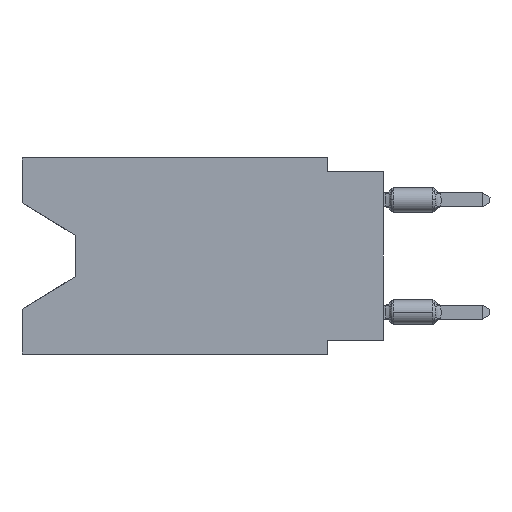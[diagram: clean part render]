
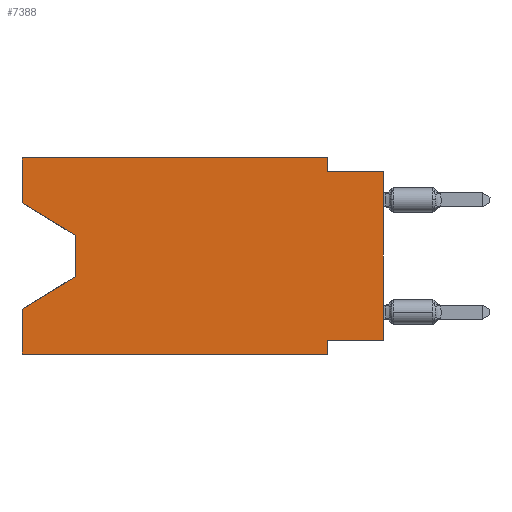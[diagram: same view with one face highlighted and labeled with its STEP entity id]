
A CAD part, left-side view. The second image highlights one B-rep face of the part: STEP entity #7388.
In plain terms, the highlighted planar face has unit normal (-1, 0, 0).
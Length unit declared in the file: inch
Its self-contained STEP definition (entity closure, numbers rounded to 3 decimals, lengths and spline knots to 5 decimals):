
#37 = FACE_OUTER_BOUND ( 'NONE', #12232, .T. ) ;
#571 = VERTEX_POINT ( 'NONE', #2002 ) ;
#631 = CARTESIAN_POINT ( 'NONE',  ( 0., 0., -0.025 ) ) ;
#849 = LINE ( 'NONE', #13853, #3731 ) ;
#866 = DIRECTION ( 'NONE',  ( 0., 0., 1. ) ) ;
#1081 = AXIS2_PLACEMENT_3D ( 'NONE', #1236, #5562, #4346 ) ;
#1091 = VECTOR ( 'NONE', #2342, 39.37008 ) ;
#1120 = DIRECTION ( 'NONE',  ( 0., -0.855, -0.519 ) ) ;
#1163 = LINE ( 'NONE', #9508, #10827 ) ;
#1192 = CARTESIAN_POINT ( 'NONE',  ( 0., 0.1, 0. ) ) ;
#1236 = CARTESIAN_POINT ( 'NONE',  ( 0., 0.645, 0. ) ) ;
#1350 = VECTOR ( 'NONE', #2561, 39.37008 ) ;
#1513 = EDGE_CURVE ( 'NONE', #12608, #571, #4302, .T. ) ;
#1532 = CARTESIAN_POINT ( 'NONE',  ( 0., 0.645, -0.26975 ) ) ;
#2002 = CARTESIAN_POINT ( 'NONE',  ( 0., 0.55, -0.138 ) ) ;
#2152 = CARTESIAN_POINT ( 'NONE',  ( 0., 0.645, -0.35 ) ) ;
#2342 = DIRECTION ( 'NONE',  ( 0., -1., 0. ) ) ;
#2561 = DIRECTION ( 'NONE',  ( 0., -1., 0. ) ) ;
#2607 = VERTEX_POINT ( 'NONE', #5348 ) ;
#2812 = CARTESIAN_POINT ( 'NONE',  ( 0., 0.645, 0. ) ) ;
#3357 = VERTEX_POINT ( 'NONE', #7820 ) ;
#3711 = VECTOR ( 'NONE', #9284, 39.37008 ) ;
#3731 = VECTOR ( 'NONE', #4169, 39.37008 ) ;
#3754 = ORIENTED_EDGE ( 'NONE', *, *, #10575, .T. ) ;
#3877 = VERTEX_POINT ( 'NONE', #5956 ) ;
#4086 = ORIENTED_EDGE ( 'NONE', *, *, #13503, .F. ) ;
#4095 = VERTEX_POINT ( 'NONE', #4251 ) ;
#4169 = DIRECTION ( 'NONE',  ( 0., 1., 0. ) ) ;
#4251 = CARTESIAN_POINT ( 'NONE',  ( 0., 0.645, -0.35 ) ) ;
#4302 = LINE ( 'NONE', #8616, #10107 ) ;
#4336 = LINE ( 'NONE', #2152, #10252 ) ;
#4346 = DIRECTION ( 'NONE',  ( 0., 0., -1. ) ) ;
#4405 = VECTOR ( 'NONE', #9842, 39.37008 ) ;
#4422 = EDGE_CURVE ( 'NONE', #4095, #4780, #12509, .T. ) ;
#4452 = VERTEX_POINT ( 'NONE', #6669 ) ;
#4695 = EDGE_CURVE ( 'NONE', #4452, #2607, #849, .T. ) ;
#4780 = VERTEX_POINT ( 'NONE', #1532 ) ;
#4797 = ORIENTED_EDGE ( 'NONE', *, *, #4695, .F. ) ;
#4812 = ORIENTED_EDGE ( 'NONE', *, *, #5375, .F. ) ;
#4821 = VERTEX_POINT ( 'NONE', #8946 ) ;
#4937 = ORIENTED_EDGE ( 'NONE', *, *, #6341, .T. ) ;
#4971 = CARTESIAN_POINT ( 'NONE',  ( 0., 0.645, 0. ) ) ;
#5242 = EDGE_CURVE ( 'NONE', #4452, #3357, #7875, .T. ) ;
#5348 = CARTESIAN_POINT ( 'NONE',  ( 0., 0.1, -0.325 ) ) ;
#5375 = EDGE_CURVE ( 'NONE', #12608, #5880, #10342, .T. ) ;
#5435 = DIRECTION ( 'NONE',  ( 0., 0., -1. ) ) ;
#5477 = DIRECTION ( 'NONE',  ( 0., 0., -1. ) ) ;
#5562 = DIRECTION ( 'NONE',  ( 1., 0., 0. ) ) ;
#5565 = ORIENTED_EDGE ( 'NONE', *, *, #8524, .F. ) ;
#5606 = LINE ( 'NONE', #12319, #5875 ) ;
#5810 = ORIENTED_EDGE ( 'NONE', *, *, #12547, .T. ) ;
#5875 = VECTOR ( 'NONE', #12038, 39.37008 ) ;
#5880 = VERTEX_POINT ( 'NONE', #8700 ) ;
#5956 = CARTESIAN_POINT ( 'NONE',  ( 0., 0.1, 0. ) ) ;
#5979 = CARTESIAN_POINT ( 'NONE',  ( 0., 0.55, -0.212 ) ) ;
#6323 = CARTESIAN_POINT ( 'NONE',  ( 0., 0.1, -0.35 ) ) ;
#6341 = EDGE_CURVE ( 'NONE', #571, #11213, #5606, .T. ) ;
#6587 = ORIENTED_EDGE ( 'NONE', *, *, #1513, .T. ) ;
#6669 = CARTESIAN_POINT ( 'NONE',  ( 0., 0., -0.325 ) ) ;
#7020 = ORIENTED_EDGE ( 'NONE', *, *, #7971, .F. ) ;
#7388 = ADVANCED_FACE ( 'NONE', ( #37 ), #10646, .F. ) ;
#7820 = CARTESIAN_POINT ( 'NONE',  ( 0., 0., -0.025 ) ) ;
#7867 = VERTEX_POINT ( 'NONE', #6323 ) ;
#7875 = LINE ( 'NONE', #8427, #13649 ) ;
#7940 = LINE ( 'NONE', #8862, #1350 ) ;
#7971 = EDGE_CURVE ( 'NONE', #4821, #3357, #13505, .T. ) ;
#8427 = CARTESIAN_POINT ( 'NONE',  ( 0., 0., 0. ) ) ;
#8524 = EDGE_CURVE ( 'NONE', #2607, #7867, #1163, .T. ) ;
#8616 = CARTESIAN_POINT ( 'NONE',  ( 0., 0.645, -0.08025 ) ) ;
#8673 = EDGE_CURVE ( 'NONE', #5880, #3877, #7940, .T. ) ;
#8700 = CARTESIAN_POINT ( 'NONE',  ( 0., 0.645, 0. ) ) ;
#8760 = LINE ( 'NONE', #1192, #10063 ) ;
#8823 = DIRECTION ( 'NONE',  ( 0., 0.855, -0.519 ) ) ;
#8862 = CARTESIAN_POINT ( 'NONE',  ( 0., 0.645, 0. ) ) ;
#8946 = CARTESIAN_POINT ( 'NONE',  ( 0., 0.1, -0.025 ) ) ;
#9284 = DIRECTION ( 'NONE',  ( 0., 0., 1. ) ) ;
#9369 = ORIENTED_EDGE ( 'NONE', *, *, #4422, .F. ) ;
#9503 = CARTESIAN_POINT ( 'NONE',  ( 0., 0.645, -0.08025 ) ) ;
#9508 = CARTESIAN_POINT ( 'NONE',  ( 0., 0.1, -0.35 ) ) ;
#9842 = DIRECTION ( 'NONE',  ( 0., 0., 1. ) ) ;
#9955 = CARTESIAN_POINT ( 'NONE',  ( 0., 0.55, -0.212 ) ) ;
#10063 = VECTOR ( 'NONE', #5435, 39.37008 ) ;
#10107 = VECTOR ( 'NONE', #1120, 39.37008 ) ;
#10252 = VECTOR ( 'NONE', #12899, 39.37008 ) ;
#10342 = LINE ( 'NONE', #4971, #3711 ) ;
#10575 = EDGE_CURVE ( 'NONE', #11213, #4780, #12083, .T. ) ;
#10646 = PLANE ( 'NONE',  #1081 ) ;
#10658 = ORIENTED_EDGE ( 'NONE', *, *, #8673, .F. ) ;
#10827 = VECTOR ( 'NONE', #5477, 39.37008 ) ;
#11213 = VERTEX_POINT ( 'NONE', #5979 ) ;
#11498 = ORIENTED_EDGE ( 'NONE', *, *, #5242, .T. ) ;
#12038 = DIRECTION ( 'NONE',  ( 0., 0., -1. ) ) ;
#12083 = LINE ( 'NONE', #9955, #12856 ) ;
#12232 = EDGE_LOOP ( 'NONE', ( #6587, #4937, #3754, #9369, #5810, #5565, #4797, #11498, #7020, #4086, #10658, #4812 ) ) ;
#12319 = CARTESIAN_POINT ( 'NONE',  ( 0., 0.55, -0.138 ) ) ;
#12509 = LINE ( 'NONE', #2812, #4405 ) ;
#12547 = EDGE_CURVE ( 'NONE', #4095, #7867, #4336, .T. ) ;
#12608 = VERTEX_POINT ( 'NONE', #9503 ) ;
#12856 = VECTOR ( 'NONE', #8823, 39.37008 ) ;
#12899 = DIRECTION ( 'NONE',  ( 0., -1., 0. ) ) ;
#13503 = EDGE_CURVE ( 'NONE', #3877, #4821, #8760, .T. ) ;
#13505 = LINE ( 'NONE', #631, #1091 ) ;
#13649 = VECTOR ( 'NONE', #866, 39.37008 ) ;
#13853 = CARTESIAN_POINT ( 'NONE',  ( 0., 0., -0.325 ) ) ;
